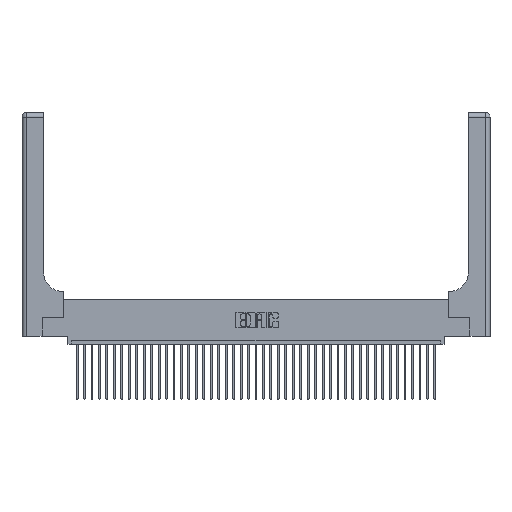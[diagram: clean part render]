
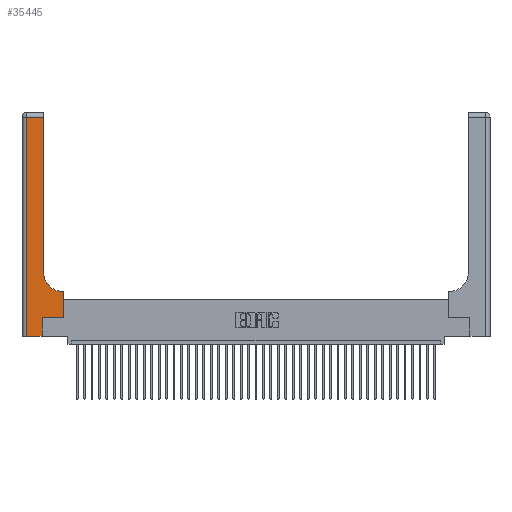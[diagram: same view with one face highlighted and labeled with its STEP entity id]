
A CAD part, top view. The second image highlights one B-rep face of the part: STEP entity #35445.
In plain terms, the highlighted planar face has unit normal (0, 0, 1).
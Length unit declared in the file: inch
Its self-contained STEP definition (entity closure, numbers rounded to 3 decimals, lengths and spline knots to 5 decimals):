
#676 = DIRECTION ( 'NONE',  ( -1., 0., 0. ) ) ;
#1447 = DIRECTION ( 'NONE',  ( 0., 1., 0. ) ) ;
#2307 = DIRECTION ( 'NONE',  ( -1., 0., 0. ) ) ;
#2756 = CARTESIAN_POINT ( 'NONE',  ( 0.06, 0., 0.37 ) ) ;
#4787 = DIRECTION ( 'NONE',  ( 1., 0., 0. ) ) ;
#5531 = CARTESIAN_POINT ( 'NONE',  ( 0., 0., 0.37 ) ) ;
#6098 = LINE ( 'NONE', #16213, #21561 ) ;
#6384 = CARTESIAN_POINT ( 'NONE',  ( 0.06, 2.94, 0.37 ) ) ;
#6996 = EDGE_CURVE ( 'NONE', #25046, #14032, #35165, .T. ) ;
#7562 = EDGE_CURVE ( 'NONE', #24514, #16282, #21236, .T. ) ;
#7678 = EDGE_CURVE ( 'NONE', #34965, #25046, #38614, .T. ) ;
#8496 = VERTEX_POINT ( 'NONE', #35689 ) ;
#8713 = CARTESIAN_POINT ( 'NONE',  ( 0.5415, 0.6, 0.37 ) ) ;
#9091 = EDGE_CURVE ( 'NONE', #40051, #24514, #6098, .T. ) ;
#10287 = ORIENTED_EDGE ( 'NONE', *, *, #17238, .T. ) ;
#10389 = EDGE_LOOP ( 'NONE', ( #10287, #14149, #20970, #35391, #22891, #26830, #31878, #40618, #29905 ) ) ;
#11180 = VECTOR ( 'NONE', #11822, 39.37008 ) ;
#11822 = DIRECTION ( 'NONE',  ( 1., 0., 0. ) ) ;
#12050 = DIRECTION ( 'NONE',  ( 0., -1., 0. ) ) ;
#12131 = VECTOR ( 'NONE', #30896, 39.37008 ) ;
#13644 = DIRECTION ( 'NONE',  ( 0., 0., -1. ) ) ;
#14032 = VERTEX_POINT ( 'NONE', #14394 ) ;
#14149 = ORIENTED_EDGE ( 'NONE', *, *, #17507, .T. ) ;
#14394 = CARTESIAN_POINT ( 'NONE',  ( 0.5585, 0.25, 0.37 ) ) ;
#14754 = CARTESIAN_POINT ( 'NONE',  ( 0.5585, 0.25, 0.37 ) ) ;
#16213 = CARTESIAN_POINT ( 'NONE',  ( 0.2915, 0.6, 0.37 ) ) ;
#16282 = VERTEX_POINT ( 'NONE', #19995 ) ;
#17163 = CARTESIAN_POINT ( 'NONE',  ( 0., 3., 0.37 ) ) ;
#17238 = EDGE_CURVE ( 'NONE', #16282, #8496, #22723, .T. ) ;
#17373 = LINE ( 'NONE', #29357, #38274 ) ;
#17507 = EDGE_CURVE ( 'NONE', #8496, #25726, #17373, .T. ) ;
#17650 = CARTESIAN_POINT ( 'NONE',  ( 0.2915, 3., 0.37 ) ) ;
#18968 = EDGE_CURVE ( 'NONE', #25726, #19492, #26568, .T. ) ;
#19125 = LINE ( 'NONE', #14754, #12131 ) ;
#19412 = EDGE_CURVE ( 'NONE', #19492, #34965, #28122, .T. ) ;
#19492 = VERTEX_POINT ( 'NONE', #2756 ) ;
#19995 = CARTESIAN_POINT ( 'NONE',  ( 0.2915, 0.85, 0.37 ) ) ;
#20970 = ORIENTED_EDGE ( 'NONE', *, *, #18968, .T. ) ;
#21031 = AXIS2_PLACEMENT_3D ( 'NONE', #34391, #40842, #21713 ) ;
#21229 = VECTOR ( 'NONE', #4787, 39.37008 ) ;
#21236 = CIRCLE ( 'NONE', #21031, 0.25 ) ;
#21561 = VECTOR ( 'NONE', #2307, 39.37008 ) ;
#21713 = DIRECTION ( 'NONE',  ( 1., 0., 0. ) ) ;
#22723 = LINE ( 'NONE', #17650, #26733 ) ;
#22891 = ORIENTED_EDGE ( 'NONE', *, *, #7678, .T. ) ;
#23326 = AXIS2_PLACEMENT_3D ( 'NONE', #17163, #13644, #35912 ) ;
#23390 = CARTESIAN_POINT ( 'NONE',  ( 0.5585, 0.6, 0.37 ) ) ;
#23525 = CARTESIAN_POINT ( 'NONE',  ( 0.269, 0., 0.37 ) ) ;
#23839 = CARTESIAN_POINT ( 'NONE',  ( 0.269, 0.25, 0.37 ) ) ;
#24514 = VERTEX_POINT ( 'NONE', #8713 ) ;
#25046 = VERTEX_POINT ( 'NONE', #38595 ) ;
#25726 = VERTEX_POINT ( 'NONE', #6384 ) ;
#26535 = PLANE ( 'NONE',  #23326 ) ;
#26568 = LINE ( 'NONE', #40908, #33614 ) ;
#26733 = VECTOR ( 'NONE', #1447, 39.37008 ) ;
#26830 = ORIENTED_EDGE ( 'NONE', *, *, #6996, .T. ) ;
#28122 = LINE ( 'NONE', #5531, #11180 ) ;
#28830 = EDGE_CURVE ( 'NONE', #14032, #40051, #19125, .T. ) ;
#29085 = DIRECTION ( 'NONE',  ( 0., 1., 0. ) ) ;
#29357 = CARTESIAN_POINT ( 'NONE',  ( 0., 2.94, 0.37 ) ) ;
#29905 = ORIENTED_EDGE ( 'NONE', *, *, #7562, .T. ) ;
#30896 = DIRECTION ( 'NONE',  ( 0., 1., 0. ) ) ;
#31878 = ORIENTED_EDGE ( 'NONE', *, *, #28830, .T. ) ;
#33587 = CARTESIAN_POINT ( 'NONE',  ( 0.269, 0., 0.37 ) ) ;
#33614 = VECTOR ( 'NONE', #12050, 39.37008 ) ;
#34391 = CARTESIAN_POINT ( 'NONE',  ( 0.5415, 0.85, 0.37 ) ) ;
#34965 = VERTEX_POINT ( 'NONE', #33587 ) ;
#35165 = LINE ( 'NONE', #23839, #21229 ) ;
#35391 = ORIENTED_EDGE ( 'NONE', *, *, #19412, .T. ) ;
#35445 = ADVANCED_FACE ( 'NONE', ( #38617 ), #26535, .F. ) ;
#35689 = CARTESIAN_POINT ( 'NONE',  ( 0.2915, 2.94, 0.37 ) ) ;
#35912 = DIRECTION ( 'NONE',  ( -1., 0., 0. ) ) ;
#37658 = VECTOR ( 'NONE', #29085, 39.37008 ) ;
#38274 = VECTOR ( 'NONE', #676, 39.37008 ) ;
#38595 = CARTESIAN_POINT ( 'NONE',  ( 0.269, 0.25, 0.37 ) ) ;
#38614 = LINE ( 'NONE', #23525, #37658 ) ;
#38617 = FACE_OUTER_BOUND ( 'NONE', #10389, .T. ) ;
#40051 = VERTEX_POINT ( 'NONE', #23390 ) ;
#40618 = ORIENTED_EDGE ( 'NONE', *, *, #9091, .T. ) ;
#40842 = DIRECTION ( 'NONE',  ( 0., 0., -1. ) ) ;
#40908 = CARTESIAN_POINT ( 'NONE',  ( 0.06, 3., 0.37 ) ) ;
